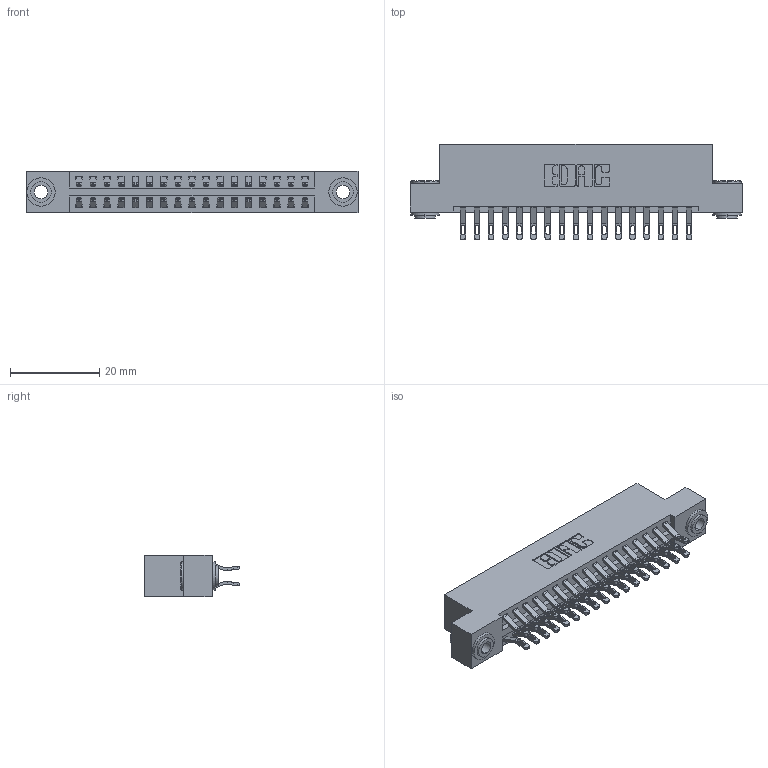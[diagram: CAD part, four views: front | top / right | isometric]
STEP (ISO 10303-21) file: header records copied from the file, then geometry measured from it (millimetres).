
FILE_DESCRIPTION (( 'STEP AP203' ), '1' );
FILE_NAME ('396-034-555-203.STEP', '2018-09-06T01:14:59', ( '' ), ( '' ), 'SwSTEP 2.0', 'SolidWorks 2016', '' );
FILE_SCHEMA (( 'CONFIG_CONTROL_DESIGN' ));
Length unit declared in the file: inch
Products named in the file (4): 346 Part_Flush Mounting Lugs - 0.156 Dia-TH; 345-292-001_555 Tail; 345-250-002_345-250-002-102; 396-034-555-203
Assembly tree (37 placements, depth 2):
  396-034-555-203
    346 Part_Flush Mounting Lugs - 0.156 Dia-TH
    345-292-001_555 Tail  x34
    345-250-002_345-250-002-102  x2
Bounding box: 74.55 x 21.46 x 9.4 mm (x, y, z)
Volume: 7193.3 mm3; surface area: 10060.4 mm2
Topology: 37 solids, 37 shells, 2132 faces, 6627 edges, 4414 vertices
Faces by surface type: plane 1208, cylinder 916, cone 8
Entity records: 15436 total; most frequent: CARTESIAN_POINT 2589, ORIENTED_EDGE 2486, DIRECTION 2333, EDGE_CURVE 1243, VECTOR 999, LINE 999, VERTEX_POINT 826, AXIS2_PLACEMENT_3D 667
